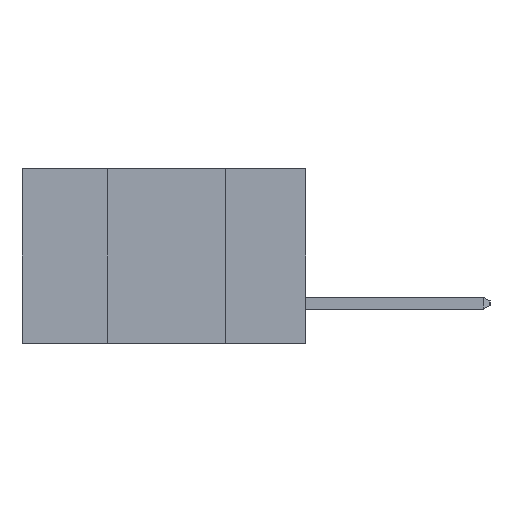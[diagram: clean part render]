
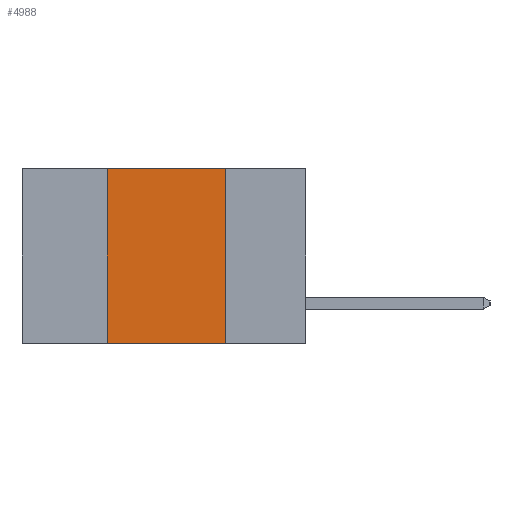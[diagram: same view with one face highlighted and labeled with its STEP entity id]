
A CAD part, left-side view. The second image highlights one B-rep face of the part: STEP entity #4988.
In plain terms, the highlighted planar face has unit normal (-1, 0, 0).
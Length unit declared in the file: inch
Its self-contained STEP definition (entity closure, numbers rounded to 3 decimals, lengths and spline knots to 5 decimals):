
#3 = DIRECTION ( 'NONE',  ( 0., 0., 1. ) ) ;
#27 = CARTESIAN_POINT ( 'NONE',  ( 0., 0.42, -0.37 ) ) ;
#502 = DIRECTION ( 'NONE',  ( 0., 0., -1. ) ) ;
#536 = LINE ( 'NONE', #585, #7571 ) ;
#585 = CARTESIAN_POINT ( 'NONE',  ( 0., 0.17, -0.37 ) ) ;
#2740 = VERTEX_POINT ( 'NONE', #7116 ) ;
#2795 = VERTEX_POINT ( 'NONE', #5594 ) ;
#2928 = AXIS2_PLACEMENT_3D ( 'NONE', #7109, #7101, #7094 ) ;
#3420 = VECTOR ( 'NONE', #5661, 39.37008 ) ;
#3489 = VECTOR ( 'NONE', #7576, 39.37008 ) ;
#3590 = EDGE_CURVE ( 'NONE', #2795, #8650, #536, .T. ) ;
#3631 = FACE_OUTER_BOUND ( 'NONE', #8314, .T. ) ;
#4073 = EDGE_CURVE ( 'NONE', #8548, #2795, #8864, .T. ) ;
#4230 = CARTESIAN_POINT ( 'NONE',  ( 0., 0.42, 0. ) ) ;
#4296 = CARTESIAN_POINT ( 'NONE',  ( 0., 0.6, -0.37 ) ) ;
#4638 = ORIENTED_EDGE ( 'NONE', *, *, #3590, .F. ) ;
#4988 = ADVANCED_FACE ( 'NONE', ( #3631 ), #7256, .F. ) ;
#5411 = CARTESIAN_POINT ( 'NONE',  ( 0., 0.6, 0. ) ) ;
#5505 = EDGE_CURVE ( 'NONE', #2740, #8548, #5842, .T. ) ;
#5594 = CARTESIAN_POINT ( 'NONE',  ( 0., 0.17, 0. ) ) ;
#5661 = DIRECTION ( 'NONE',  ( 0., -1., 0. ) ) ;
#5842 = LINE ( 'NONE', #27, #7436 ) ;
#5968 = EDGE_CURVE ( 'NONE', #2740, #8650, #8739, .T. ) ;
#6169 = ORIENTED_EDGE ( 'NONE', *, *, #5968, .T. ) ;
#6278 = ORIENTED_EDGE ( 'NONE', *, *, #5505, .F. ) ;
#7094 = DIRECTION ( 'NONE',  ( 0., 0., -1. ) ) ;
#7101 = DIRECTION ( 'NONE',  ( 1., 0., 0. ) ) ;
#7109 = CARTESIAN_POINT ( 'NONE',  ( 0., 0.6, 0. ) ) ;
#7116 = CARTESIAN_POINT ( 'NONE',  ( 0., 0.42, -0.37 ) ) ;
#7256 = PLANE ( 'NONE',  #2928 ) ;
#7436 = VECTOR ( 'NONE', #3, 39.37008 ) ;
#7571 = VECTOR ( 'NONE', #502, 39.37008 ) ;
#7576 = DIRECTION ( 'NONE',  ( 0., -1., 0. ) ) ;
#8062 = ORIENTED_EDGE ( 'NONE', *, *, #4073, .F. ) ;
#8314 = EDGE_LOOP ( 'NONE', ( #4638, #8062, #6278, #6169 ) ) ;
#8545 = CARTESIAN_POINT ( 'NONE',  ( 0., 0.17, -0.37 ) ) ;
#8548 = VERTEX_POINT ( 'NONE', #4230 ) ;
#8650 = VERTEX_POINT ( 'NONE', #8545 ) ;
#8739 = LINE ( 'NONE', #4296, #3489 ) ;
#8864 = LINE ( 'NONE', #5411, #3420 ) ;
